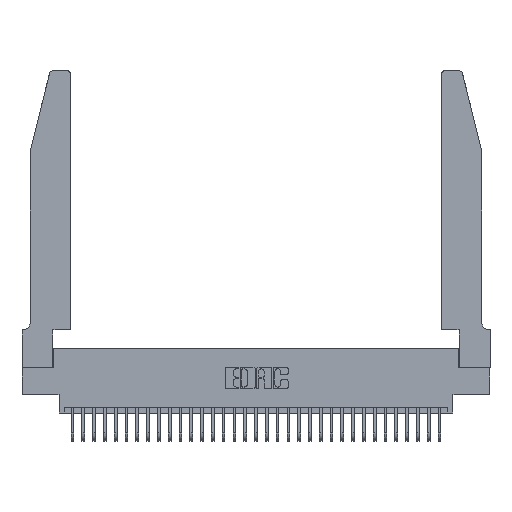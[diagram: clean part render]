
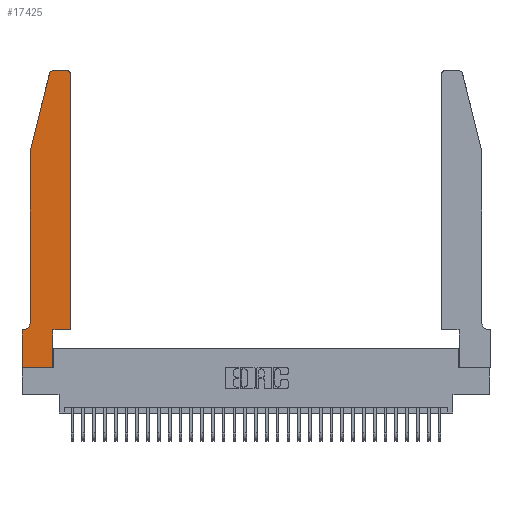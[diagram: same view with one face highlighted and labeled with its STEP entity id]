
A CAD part, top view. The second image highlights one B-rep face of the part: STEP entity #17425.
In plain terms, the highlighted planar face has unit normal (0, 0, 1).
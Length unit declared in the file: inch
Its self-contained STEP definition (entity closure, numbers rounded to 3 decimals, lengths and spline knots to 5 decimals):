
#755 = CARTESIAN_POINT ( 'NONE',  ( 0., 0.35, 0.37 ) ) ;
#1044 = DIRECTION ( 'NONE',  ( 0., -1., 0. ) ) ;
#1261 = DIRECTION ( 'NONE',  ( 1., 0., 0. ) ) ;
#1479 = VERTEX_POINT ( 'NONE', #23988 ) ;
#1872 = CARTESIAN_POINT ( 'NONE',  ( 0.2865, 0., 0.37 ) ) ;
#2237 = EDGE_CURVE ( 'NONE', #30919, #28989, #7527, .T. ) ;
#2342 = VERTEX_POINT ( 'NONE', #10398 ) ;
#2579 = ORIENTED_EDGE ( 'NONE', *, *, #18917, .T. ) ;
#3628 = DIRECTION ( 'NONE',  ( 0., 1., 0. ) ) ;
#3691 = VECTOR ( 'NONE', #7023, 39.37008 ) ;
#4958 = PLANE ( 'NONE',  #13654 ) ;
#5032 = LINE ( 'NONE', #30934, #17514 ) ;
#5232 = VERTEX_POINT ( 'NONE', #26638 ) ;
#5507 = VERTEX_POINT ( 'NONE', #755 ) ;
#5827 = CARTESIAN_POINT ( 'NONE',  ( 0.4505, 0.35, 0.37 ) ) ;
#7023 = DIRECTION ( 'NONE',  ( 1., 0., 0. ) ) ;
#7451 = EDGE_CURVE ( 'NONE', #22866, #28056, #16960, .T. ) ;
#7477 = DIRECTION ( 'NONE',  ( 1., 0., 0. ) ) ;
#7527 = CIRCLE ( 'NONE', #21707, 0.03 ) ;
#8319 = DIRECTION ( 'NONE',  ( 1., 0., 0. ) ) ;
#9271 = CARTESIAN_POINT ( 'NONE',  ( 0.2865, 0.35, 0.37 ) ) ;
#9639 = VECTOR ( 'NONE', #14576, 39.37008 ) ;
#9955 = DIRECTION ( 'NONE',  ( 0., 0., -1. ) ) ;
#10398 = CARTESIAN_POINT ( 'NONE',  ( 0.4205, 2.75, 0.37 ) ) ;
#11044 = DIRECTION ( 'NONE',  ( -0.239, -0.971, 0. ) ) ;
#11100 = CARTESIAN_POINT ( 'NONE',  ( 0.0755, 0.42, 0.37 ) ) ;
#11309 = LINE ( 'NONE', #5827, #30384 ) ;
#11322 = CARTESIAN_POINT ( 'NONE',  ( 0., 0., 0.37 ) ) ;
#11324 = CARTESIAN_POINT ( 'NONE',  ( 0.4505, 2.72, 0.37 ) ) ;
#12040 = CARTESIAN_POINT ( 'NONE',  ( 0., 0., 0.37 ) ) ;
#12129 = ORIENTED_EDGE ( 'NONE', *, *, #16268, .T. ) ;
#12153 = DIRECTION ( 'NONE',  ( 0., 0., 1. ) ) ;
#12935 = CIRCLE ( 'NONE', #26152, 0.07 ) ;
#13020 = VERTEX_POINT ( 'NONE', #9271 ) ;
#13554 = EDGE_CURVE ( 'NONE', #31850, #2342, #19972, .T. ) ;
#13654 = AXIS2_PLACEMENT_3D ( 'NONE', #32165, #22429, #7477 ) ;
#14131 = ORIENTED_EDGE ( 'NONE', *, *, #21178, .T. ) ;
#14576 = DIRECTION ( 'NONE',  ( -1., 0., 0. ) ) ;
#14776 = ORIENTED_EDGE ( 'NONE', *, *, #7451, .T. ) ;
#14908 = ORIENTED_EDGE ( 'NONE', *, *, #13554, .T. ) ;
#15049 = EDGE_CURVE ( 'NONE', #28056, #13020, #23959, .T. ) ;
#15255 = ORIENTED_EDGE ( 'NONE', *, *, #2237, .T. ) ;
#15895 = EDGE_CURVE ( 'NONE', #5232, #29361, #30481, .T. ) ;
#15997 = FACE_OUTER_BOUND ( 'NONE', #30699, .T. ) ;
#16092 = CARTESIAN_POINT ( 'NONE',  ( 0.4505, 0.35, 0.37 ) ) ;
#16098 = VERTEX_POINT ( 'NONE', #26787 ) ;
#16238 = DIRECTION ( 'NONE',  ( 0., 0., 1. ) ) ;
#16268 = EDGE_CURVE ( 'NONE', #29361, #1479, #12935, .T. ) ;
#16275 = LINE ( 'NONE', #11322, #23680 ) ;
#16480 = VECTOR ( 'NONE', #1044, 39.37008 ) ;
#16689 = ORIENTED_EDGE ( 'NONE', *, *, #27878, .T. ) ;
#16960 = LINE ( 'NONE', #12040, #3691 ) ;
#17299 = VECTOR ( 'NONE', #20155, 39.37008 ) ;
#17425 = ADVANCED_FACE ( 'NONE', ( #15997 ), #4958, .T. ) ;
#17514 = VECTOR ( 'NONE', #18532, 39.37008 ) ;
#17663 = CARTESIAN_POINT ( 'NONE',  ( 0.2865, 0.35, 0.37 ) ) ;
#17726 = AXIS2_PLACEMENT_3D ( 'NONE', #31112, #16238, #1261 ) ;
#18072 = VECTOR ( 'NONE', #3628, 39.37008 ) ;
#18483 = ORIENTED_EDGE ( 'NONE', *, *, #26113, .T. ) ;
#18493 = CARTESIAN_POINT ( 'NONE',  ( 0.0755, 2., 0.37 ) ) ;
#18532 = DIRECTION ( 'NONE',  ( -1., 0., 0. ) ) ;
#18917 = EDGE_CURVE ( 'NONE', #5507, #22866, #16275, .T. ) ;
#19299 = ORIENTED_EDGE ( 'NONE', *, *, #15895, .T. ) ;
#19972 = CIRCLE ( 'NONE', #17726, 0.03 ) ;
#20155 = DIRECTION ( 'NONE',  ( 0., 1., 0. ) ) ;
#21178 = EDGE_CURVE ( 'NONE', #2342, #30919, #22906, .T. ) ;
#21707 = AXIS2_PLACEMENT_3D ( 'NONE', #27098, #12153, #29576 ) ;
#22232 = LINE ( 'NONE', #23475, #28067 ) ;
#22429 = DIRECTION ( 'NONE',  ( 0., 0., 1. ) ) ;
#22866 = VERTEX_POINT ( 'NONE', #24268 ) ;
#22906 = LINE ( 'NONE', #31832, #9639 ) ;
#23475 = CARTESIAN_POINT ( 'NONE',  ( 0.0755, 2., 0.37 ) ) ;
#23680 = VECTOR ( 'NONE', #28759, 39.37008 ) ;
#23959 = LINE ( 'NONE', #17663, #17299 ) ;
#23988 = CARTESIAN_POINT ( 'NONE',  ( 0.0055, 0.35, 0.37 ) ) ;
#24268 = CARTESIAN_POINT ( 'NONE',  ( 0., 0., 0.37 ) ) ;
#24920 = CARTESIAN_POINT ( 'NONE',  ( 0.0055, 0.42, 0.37 ) ) ;
#25548 = EDGE_CURVE ( 'NONE', #1479, #5507, #5032, .T. ) ;
#26041 = EDGE_CURVE ( 'NONE', #13020, #16098, #11309, .T. ) ;
#26113 = EDGE_CURVE ( 'NONE', #28989, #5232, #22232, .T. ) ;
#26152 = AXIS2_PLACEMENT_3D ( 'NONE', #24920, #9955, #27419 ) ;
#26548 = ORIENTED_EDGE ( 'NONE', *, *, #15049, .T. ) ;
#26638 = CARTESIAN_POINT ( 'NONE',  ( 0.0755, 2., 0.37 ) ) ;
#26787 = CARTESIAN_POINT ( 'NONE',  ( 0.4505, 0.35, 0.37 ) ) ;
#27047 = CARTESIAN_POINT ( 'NONE',  ( 0.25487, 2.72718, 0.37 ) ) ;
#27098 = CARTESIAN_POINT ( 'NONE',  ( 0.284, 2.72, 0.37 ) ) ;
#27419 = DIRECTION ( 'NONE',  ( -1., 0., 0. ) ) ;
#27587 = CARTESIAN_POINT ( 'NONE',  ( 0.284, 2.75, 0.37 ) ) ;
#27878 = EDGE_CURVE ( 'NONE', #16098, #31850, #31310, .T. ) ;
#28056 = VERTEX_POINT ( 'NONE', #1872 ) ;
#28067 = VECTOR ( 'NONE', #11044, 39.37008 ) ;
#28759 = DIRECTION ( 'NONE',  ( 0., -1., 0. ) ) ;
#28989 = VERTEX_POINT ( 'NONE', #27047 ) ;
#29220 = ORIENTED_EDGE ( 'NONE', *, *, #25548, .T. ) ;
#29361 = VERTEX_POINT ( 'NONE', #11100 ) ;
#29576 = DIRECTION ( 'NONE',  ( 1., 0., 0. ) ) ;
#30384 = VECTOR ( 'NONE', #8319, 39.37008 ) ;
#30481 = LINE ( 'NONE', #18493, #16480 ) ;
#30699 = EDGE_LOOP ( 'NONE', ( #14131, #15255, #18483, #19299, #12129, #29220, #2579, #14776, #26548, #31573, #16689, #14908 ) ) ;
#30919 = VERTEX_POINT ( 'NONE', #27587 ) ;
#30934 = CARTESIAN_POINT ( 'NONE',  ( 0.0755, 0.35, 0.37 ) ) ;
#31112 = CARTESIAN_POINT ( 'NONE',  ( 0.4205, 2.72, 0.37 ) ) ;
#31310 = LINE ( 'NONE', #16092, #18072 ) ;
#31573 = ORIENTED_EDGE ( 'NONE', *, *, #26041, .T. ) ;
#31832 = CARTESIAN_POINT ( 'NONE',  ( 0.2605, 2.75, 0.37 ) ) ;
#31850 = VERTEX_POINT ( 'NONE', #11324 ) ;
#32165 = CARTESIAN_POINT ( 'NONE',  ( 0., 0.35, 0.37 ) ) ;
